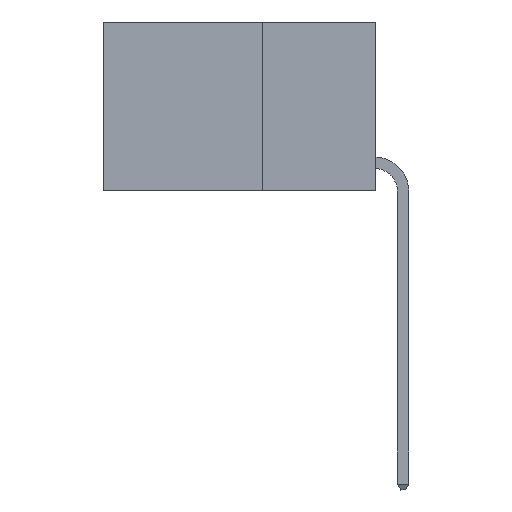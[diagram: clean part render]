
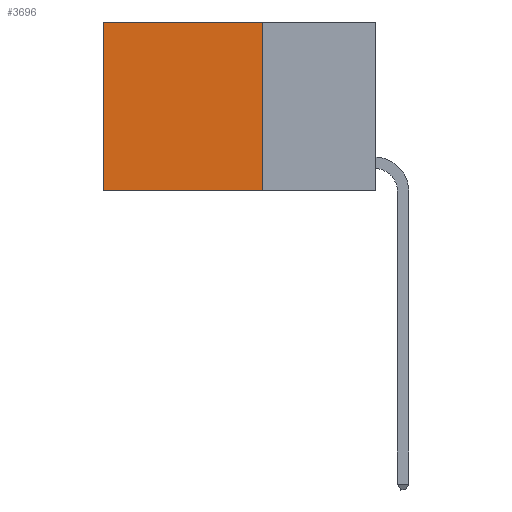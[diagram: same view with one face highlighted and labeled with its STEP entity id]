
A CAD part, left-side view. The second image highlights one B-rep face of the part: STEP entity #3696.
In plain terms, the highlighted planar face has unit normal (-1, 0, 0).
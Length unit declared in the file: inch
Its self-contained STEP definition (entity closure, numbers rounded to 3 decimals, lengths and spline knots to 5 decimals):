
#155 = ORIENTED_EDGE ( 'NONE', *, *, #4082, .F. ) ;
#1577 = CARTESIAN_POINT ( 'NONE',  ( 0.2625, 0.25, 0. ) ) ;
#1746 = EDGE_CURVE ( 'NONE', #12870, #18196, #17425, .T. ) ;
#2107 = VERTEX_POINT ( 'NONE', #14541 ) ;
#2131 = CARTESIAN_POINT ( 'NONE',  ( 0.2625, 0.25, -0.37 ) ) ;
#2301 = VERTEX_POINT ( 'NONE', #19936 ) ;
#2451 = ORIENTED_EDGE ( 'NONE', *, *, #6661, .T. ) ;
#3324 = EDGE_LOOP ( 'NONE', ( #10295, #155, #19146, #2451 ) ) ;
#3696 = ADVANCED_FACE ( 'NONE', ( #9895 ), #13661, .F. ) ;
#4082 = EDGE_CURVE ( 'NONE', #18196, #2107, #14643, .T. ) ;
#4635 = VECTOR ( 'NONE', #11113, 39.37008 ) ;
#5638 = DIRECTION ( 'NONE',  ( 0., 0., -1. ) ) ;
#5896 = AXIS2_PLACEMENT_3D ( 'NONE', #16827, #18421, #8885 ) ;
#6661 = EDGE_CURVE ( 'NONE', #12870, #2301, #8867, .T. ) ;
#6930 = CARTESIAN_POINT ( 'NONE',  ( 0.2625, 0.6, 0. ) ) ;
#8141 = EDGE_CURVE ( 'NONE', #2301, #2107, #15313, .T. ) ;
#8165 = CARTESIAN_POINT ( 'NONE',  ( 0.2625, 0.25, 0. ) ) ;
#8867 = LINE ( 'NONE', #1577, #4635 ) ;
#8885 = DIRECTION ( 'NONE',  ( 0., 0., -1. ) ) ;
#9811 = CARTESIAN_POINT ( 'NONE',  ( 0.2625, 0.25, -0.37 ) ) ;
#9895 = FACE_OUTER_BOUND ( 'NONE', #3324, .T. ) ;
#10295 = ORIENTED_EDGE ( 'NONE', *, *, #8141, .T. ) ;
#10467 = CARTESIAN_POINT ( 'NONE',  ( 0.2625, 0.25, 0. ) ) ;
#11113 = DIRECTION ( 'NONE',  ( 0., 1., 0. ) ) ;
#12870 = VERTEX_POINT ( 'NONE', #8165 ) ;
#13293 = DIRECTION ( 'NONE',  ( 0., 1., 0. ) ) ;
#13661 = PLANE ( 'NONE',  #5896 ) ;
#13714 = VECTOR ( 'NONE', #5638, 39.37008 ) ;
#14340 = VECTOR ( 'NONE', #16500, 39.37008 ) ;
#14541 = CARTESIAN_POINT ( 'NONE',  ( 0.2625, 0.6, -0.37 ) ) ;
#14643 = LINE ( 'NONE', #2131, #19320 ) ;
#15313 = LINE ( 'NONE', #6930, #14340 ) ;
#16500 = DIRECTION ( 'NONE',  ( 0., 0., -1. ) ) ;
#16827 = CARTESIAN_POINT ( 'NONE',  ( 0.2625, 0.25, 0. ) ) ;
#17425 = LINE ( 'NONE', #10467, #13714 ) ;
#18196 = VERTEX_POINT ( 'NONE', #9811 ) ;
#18421 = DIRECTION ( 'NONE',  ( 1., 0., 0. ) ) ;
#19146 = ORIENTED_EDGE ( 'NONE', *, *, #1746, .F. ) ;
#19320 = VECTOR ( 'NONE', #13293, 39.37008 ) ;
#19936 = CARTESIAN_POINT ( 'NONE',  ( 0.2625, 0.6, 0. ) ) ;
